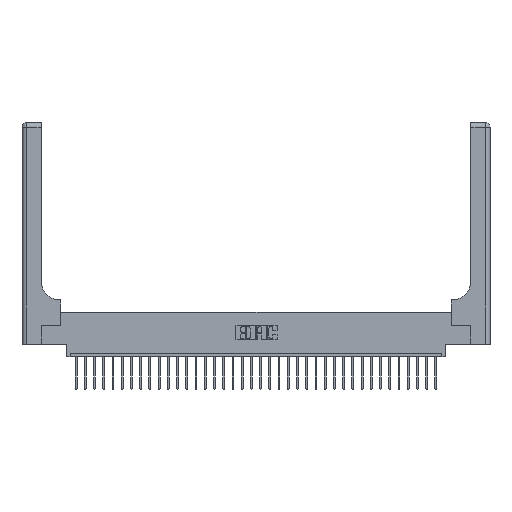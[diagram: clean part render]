
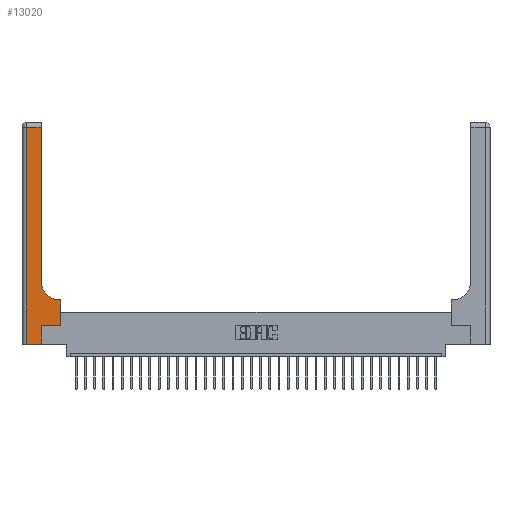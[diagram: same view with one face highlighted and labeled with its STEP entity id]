
A CAD part, top view. The second image highlights one B-rep face of the part: STEP entity #13020.
In plain terms, the highlighted planar face has unit normal (0, 0, 1).
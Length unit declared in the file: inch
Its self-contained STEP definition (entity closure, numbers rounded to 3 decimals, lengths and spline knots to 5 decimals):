
#138 = VERTEX_POINT ( 'NONE', #24466 ) ;
#678 = LINE ( 'NONE', #21999, #4695 ) ;
#739 = CARTESIAN_POINT ( 'NONE',  ( 0.51, 0.6, 0.37 ) ) ;
#1055 = EDGE_CURVE ( 'NONE', #4874, #138, #4728, .T. ) ;
#1307 = DIRECTION ( 'NONE',  ( -1., 0., 0. ) ) ;
#1384 = LINE ( 'NONE', #17710, #28593 ) ;
#2631 = DIRECTION ( 'NONE',  ( 1., 0., 0. ) ) ;
#3264 = DIRECTION ( 'NONE',  ( -1., 0., 0. ) ) ;
#3636 = DIRECTION ( 'NONE',  ( 0., -1., 0. ) ) ;
#4671 = ORIENTED_EDGE ( 'NONE', *, *, #29553, .T. ) ;
#4695 = VECTOR ( 'NONE', #8045, 39.37008 ) ;
#4728 = LINE ( 'NONE', #26070, #8422 ) ;
#4751 = DIRECTION ( 'NONE',  ( 1., 0., 0. ) ) ;
#4874 = VERTEX_POINT ( 'NONE', #25408 ) ;
#5089 = VERTEX_POINT ( 'NONE', #17647 ) ;
#5187 = ORIENTED_EDGE ( 'NONE', *, *, #11923, .T. ) ;
#5945 = DIRECTION ( 'NONE',  ( 0., 1., 0. ) ) ;
#6276 = CARTESIAN_POINT ( 'NONE',  ( 0.528, 0.25, 0.37 ) ) ;
#6305 = ORIENTED_EDGE ( 'NONE', *, *, #11031, .T. ) ;
#6608 = VECTOR ( 'NONE', #11464, 39.37008 ) ;
#7323 = VERTEX_POINT ( 'NONE', #739 ) ;
#7350 = CARTESIAN_POINT ( 'NONE',  ( 0.06, 2.94, 0.37 ) ) ;
#8045 = DIRECTION ( 'NONE',  ( 0., 1., 0. ) ) ;
#8082 = VERTEX_POINT ( 'NONE', #17045 ) ;
#8141 = CARTESIAN_POINT ( 'NONE',  ( 0.528, 0.25, 0.37 ) ) ;
#8422 = VECTOR ( 'NONE', #2631, 39.37008 ) ;
#8524 = CARTESIAN_POINT ( 'NONE',  ( 0.528, 0.6, 0.37 ) ) ;
#9204 = CARTESIAN_POINT ( 'NONE',  ( 0.51, 0.85, 0.37 ) ) ;
#9391 = CARTESIAN_POINT ( 'NONE',  ( 0.26, 0.6, 0.37 ) ) ;
#10440 = PLANE ( 'NONE',  #29160 ) ;
#10489 = DIRECTION ( 'NONE',  ( 1., 0., 0. ) ) ;
#11031 = EDGE_CURVE ( 'NONE', #5089, #13366, #23124, .T. ) ;
#11464 = DIRECTION ( 'NONE',  ( -1., 0., 0. ) ) ;
#11528 = CARTESIAN_POINT ( 'NONE',  ( 0.26, 0.85, 0.37 ) ) ;
#11923 = EDGE_CURVE ( 'NONE', #14365, #13313, #28927, .T. ) ;
#12301 = EDGE_CURVE ( 'NONE', #8082, #14365, #16077, .T. ) ;
#12590 = VECTOR ( 'NONE', #5945, 39.37008 ) ;
#12714 = CIRCLE ( 'NONE', #22730, 0.25 ) ;
#13020 = ADVANCED_FACE ( 'NONE', ( #29732 ), #10440, .F. ) ;
#13159 = VECTOR ( 'NONE', #10489, 39.37008 ) ;
#13313 = VERTEX_POINT ( 'NONE', #8524 ) ;
#13366 = VERTEX_POINT ( 'NONE', #7350 ) ;
#13914 = DIRECTION ( 'NONE',  ( 0., 0., -1. ) ) ;
#14365 = VERTEX_POINT ( 'NONE', #6276 ) ;
#14687 = VECTOR ( 'NONE', #1307, 39.37008 ) ;
#14719 = CARTESIAN_POINT ( 'NONE',  ( 0.265, 0., 0.37 ) ) ;
#14981 = VECTOR ( 'NONE', #24785, 39.37008 ) ;
#15389 = CARTESIAN_POINT ( 'NONE',  ( 0.265, 0.25, 0.37 ) ) ;
#15537 = DIRECTION ( 'NONE',  ( 0., 0., -1. ) ) ;
#16077 = LINE ( 'NONE', #15389, #13159 ) ;
#16537 = EDGE_CURVE ( 'NONE', #7323, #29136, #12714, .T. ) ;
#17045 = CARTESIAN_POINT ( 'NONE',  ( 0.265, 0.25, 0.37 ) ) ;
#17066 = ORIENTED_EDGE ( 'NONE', *, *, #12301, .T. ) ;
#17647 = CARTESIAN_POINT ( 'NONE',  ( 0.26, 2.94, 0.37 ) ) ;
#17710 = CARTESIAN_POINT ( 'NONE',  ( 0.06, 3., 0.37 ) ) ;
#18277 = EDGE_CURVE ( 'NONE', #138, #8082, #29457, .T. ) ;
#19104 = ORIENTED_EDGE ( 'NONE', *, *, #18277, .T. ) ;
#21296 = LINE ( 'NONE', #9391, #6608 ) ;
#21999 = CARTESIAN_POINT ( 'NONE',  ( 0.26, 3., 0.37 ) ) ;
#22730 = AXIS2_PLACEMENT_3D ( 'NONE', #9204, #13914, #4751 ) ;
#22872 = ORIENTED_EDGE ( 'NONE', *, *, #29869, .T. ) ;
#23124 = LINE ( 'NONE', #26890, #14687 ) ;
#23268 = EDGE_LOOP ( 'NONE', ( #22872, #6305, #4671, #30379, #19104, #17066, #5187, #25035, #29972 ) ) ;
#24466 = CARTESIAN_POINT ( 'NONE',  ( 0.265, 0., 0.37 ) ) ;
#24785 = DIRECTION ( 'NONE',  ( 0., 1., 0. ) ) ;
#25035 = ORIENTED_EDGE ( 'NONE', *, *, #28372, .T. ) ;
#25408 = CARTESIAN_POINT ( 'NONE',  ( 0.06, 0., 0.37 ) ) ;
#26070 = CARTESIAN_POINT ( 'NONE',  ( 0., 0., 0.37 ) ) ;
#26792 = CARTESIAN_POINT ( 'NONE',  ( 0., 3., 0.37 ) ) ;
#26890 = CARTESIAN_POINT ( 'NONE',  ( 0., 2.94, 0.37 ) ) ;
#28372 = EDGE_CURVE ( 'NONE', #13313, #7323, #21296, .T. ) ;
#28593 = VECTOR ( 'NONE', #3636, 39.37008 ) ;
#28927 = LINE ( 'NONE', #8141, #14981 ) ;
#29136 = VERTEX_POINT ( 'NONE', #11528 ) ;
#29160 = AXIS2_PLACEMENT_3D ( 'NONE', #26792, #15537, #3264 ) ;
#29457 = LINE ( 'NONE', #14719, #12590 ) ;
#29553 = EDGE_CURVE ( 'NONE', #13366, #4874, #1384, .T. ) ;
#29732 = FACE_OUTER_BOUND ( 'NONE', #23268, .T. ) ;
#29869 = EDGE_CURVE ( 'NONE', #29136, #5089, #678, .T. ) ;
#29972 = ORIENTED_EDGE ( 'NONE', *, *, #16537, .T. ) ;
#30379 = ORIENTED_EDGE ( 'NONE', *, *, #1055, .T. ) ;
